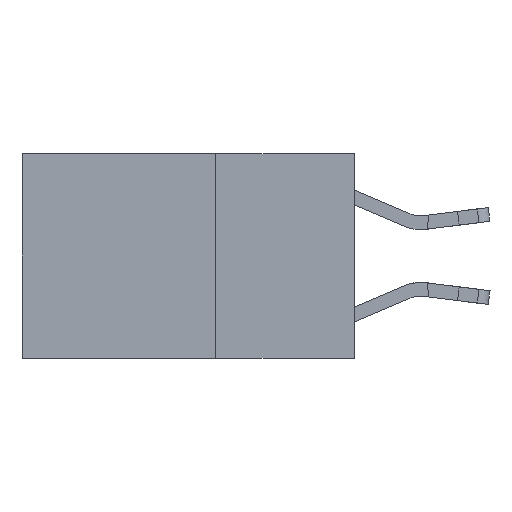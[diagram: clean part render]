
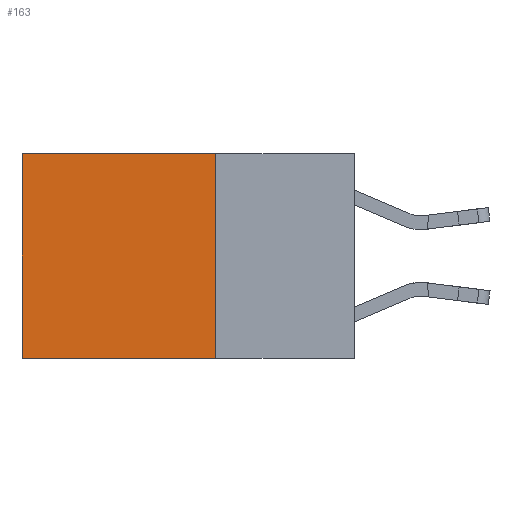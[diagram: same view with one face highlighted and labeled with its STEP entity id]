
A CAD part, left-side view. The second image highlights one B-rep face of the part: STEP entity #163.
In plain terms, the highlighted planar face has unit normal (-1, 0, 0).
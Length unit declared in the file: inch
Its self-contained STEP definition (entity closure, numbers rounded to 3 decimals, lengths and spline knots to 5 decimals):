
#163 = ADVANCED_FACE ( 'NONE', ( #17104 ), #13194, .F. ) ;
#1483 = LINE ( 'NONE', #25593, #13095 ) ;
#4061 = DIRECTION ( 'NONE',  ( 0., 0., -1. ) ) ;
#4350 = ORIENTED_EDGE ( 'NONE', *, *, #27495, .F. ) ;
#6342 = CARTESIAN_POINT ( 'NONE',  ( 0.2625, 0.25, -0.37 ) ) ;
#6854 = AXIS2_PLACEMENT_3D ( 'NONE', #28796, #17697, #4061 ) ;
#7491 = CARTESIAN_POINT ( 'NONE',  ( 0.2625, 0.25, 0. ) ) ;
#7516 = EDGE_CURVE ( 'NONE', #18943, #28829, #24467, .T. ) ;
#11912 = ORIENTED_EDGE ( 'NONE', *, *, #13403, .F. ) ;
#13095 = VECTOR ( 'NONE', #14429, 39.37008 ) ;
#13153 = DIRECTION ( 'NONE',  ( 0., 1., 0. ) ) ;
#13194 = PLANE ( 'NONE',  #6854 ) ;
#13403 = EDGE_CURVE ( 'NONE', #18943, #29004, #1483, .T. ) ;
#13972 = VECTOR ( 'NONE', #23146, 39.37008 ) ;
#14429 = DIRECTION ( 'NONE',  ( 0., 0., -1. ) ) ;
#15043 = CARTESIAN_POINT ( 'NONE',  ( 0.2625, 0.25, -0.37 ) ) ;
#15347 = VECTOR ( 'NONE', #13153, 39.37008 ) ;
#16066 = LINE ( 'NONE', #6342, #15347 ) ;
#16891 = LINE ( 'NONE', #21687, #28063 ) ;
#17104 = FACE_OUTER_BOUND ( 'NONE', #18183, .T. ) ;
#17697 = DIRECTION ( 'NONE',  ( 1., 0., 0. ) ) ;
#18183 = EDGE_LOOP ( 'NONE', ( #26273, #4350, #11912, #23812 ) ) ;
#18943 = VERTEX_POINT ( 'NONE', #23218 ) ;
#19057 = CARTESIAN_POINT ( 'NONE',  ( 0.2625, 0.6, 0. ) ) ;
#19725 = VERTEX_POINT ( 'NONE', #25881 ) ;
#21687 = CARTESIAN_POINT ( 'NONE',  ( 0.2625, 0.6, 0. ) ) ;
#23146 = DIRECTION ( 'NONE',  ( 0., 1., 0. ) ) ;
#23218 = CARTESIAN_POINT ( 'NONE',  ( 0.2625, 0.25, 0. ) ) ;
#23812 = ORIENTED_EDGE ( 'NONE', *, *, #7516, .T. ) ;
#23937 = DIRECTION ( 'NONE',  ( 0., 0., -1. ) ) ;
#24105 = EDGE_CURVE ( 'NONE', #28829, #19725, #16891, .T. ) ;
#24467 = LINE ( 'NONE', #7491, #13972 ) ;
#25593 = CARTESIAN_POINT ( 'NONE',  ( 0.2625, 0.25, 0. ) ) ;
#25881 = CARTESIAN_POINT ( 'NONE',  ( 0.2625, 0.6, -0.37 ) ) ;
#26273 = ORIENTED_EDGE ( 'NONE', *, *, #24105, .T. ) ;
#27495 = EDGE_CURVE ( 'NONE', #29004, #19725, #16066, .T. ) ;
#28063 = VECTOR ( 'NONE', #23937, 39.37008 ) ;
#28796 = CARTESIAN_POINT ( 'NONE',  ( 0.2625, 0.25, 0. ) ) ;
#28829 = VERTEX_POINT ( 'NONE', #19057 ) ;
#29004 = VERTEX_POINT ( 'NONE', #15043 ) ;
